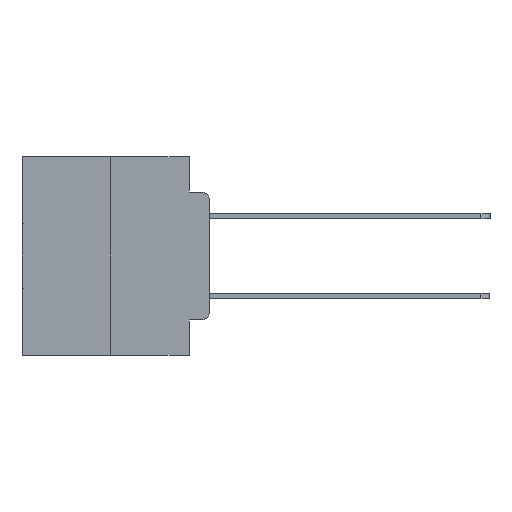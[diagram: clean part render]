
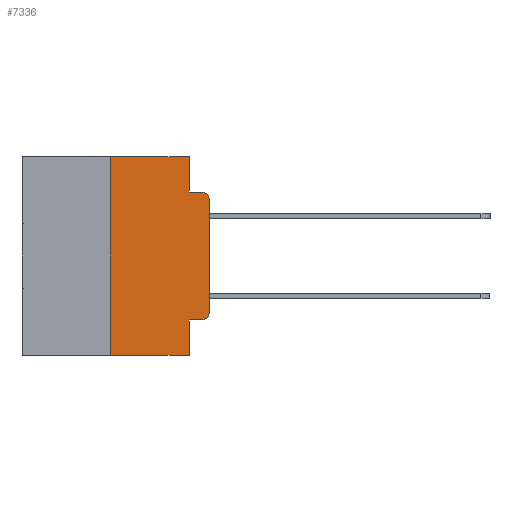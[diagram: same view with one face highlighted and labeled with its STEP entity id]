
A CAD part, left-side view. The second image highlights one B-rep face of the part: STEP entity #7336.
In plain terms, the highlighted planar face has unit normal (-1, 0, 0).
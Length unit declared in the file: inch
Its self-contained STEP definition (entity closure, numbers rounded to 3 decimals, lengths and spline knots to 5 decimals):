
#680 = CARTESIAN_POINT ( 'NONE',  ( 0., 0., -0.3915 ) ) ;
#836 = EDGE_CURVE ( 'NONE', #3411, #23348, #25860, .T. ) ;
#1466 = VECTOR ( 'NONE', #19686, 39.37008 ) ;
#1723 = ORIENTED_EDGE ( 'NONE', *, *, #10384, .T. ) ;
#2274 = EDGE_CURVE ( 'NONE', #13589, #26955, #28338, .T. ) ;
#2827 = CARTESIAN_POINT ( 'NONE',  ( 0., 0.051, 0. ) ) ;
#3411 = VERTEX_POINT ( 'NONE', #680 ) ;
#3655 = CARTESIAN_POINT ( 'NONE',  ( 0., 0.051, 0. ) ) ;
#3958 = CARTESIAN_POINT ( 'NONE',  ( 0., 0.051, -0.4115 ) ) ;
#4455 = DIRECTION ( 'NONE',  ( 0., 0., 1. ) ) ;
#5189 = DIRECTION ( 'NONE',  ( 0., 0., -1. ) ) ;
#5257 = CARTESIAN_POINT ( 'NONE',  ( 0., 0.051, 0. ) ) ;
#5335 = EDGE_CURVE ( 'NONE', #13589, #10760, #19099, .T. ) ;
#5661 = VECTOR ( 'NONE', #10762, 39.37008 ) ;
#5705 = CARTESIAN_POINT ( 'NONE',  ( 0., 0.051, -0.4115 ) ) ;
#6763 = EDGE_LOOP ( 'NONE', ( #10956, #25575, #13891, #9079, #10592, #19781, #1723, #22720, #28891, #23446 ) ) ;
#7017 = VECTOR ( 'NONE', #26369, 39.37008 ) ;
#7336 = ADVANCED_FACE ( 'NONE', ( #27312 ), #27479, .F. ) ;
#7670 = EDGE_CURVE ( 'NONE', #22380, #28418, #8952, .T. ) ;
#8102 = CARTESIAN_POINT ( 'NONE',  ( 0., 0.051, -0.0885 ) ) ;
#8650 = AXIS2_PLACEMENT_3D ( 'NONE', #10278, #26633, #12661 ) ;
#8952 = LINE ( 'NONE', #2827, #24745 ) ;
#9079 = ORIENTED_EDGE ( 'NONE', *, *, #7670, .F. ) ;
#9425 = LINE ( 'NONE', #26727, #21212 ) ;
#10012 = CARTESIAN_POINT ( 'NONE',  ( 0., 0.051, -0.0885 ) ) ;
#10278 = CARTESIAN_POINT ( 'NONE',  ( 0., 0.02, -0.3915 ) ) ;
#10384 = EDGE_CURVE ( 'NONE', #14808, #26955, #30435, .T. ) ;
#10592 = ORIENTED_EDGE ( 'NONE', *, *, #23770, .F. ) ;
#10760 = VERTEX_POINT ( 'NONE', #23239 ) ;
#10762 = DIRECTION ( 'NONE',  ( 0., 0., 1. ) ) ;
#10799 = CARTESIAN_POINT ( 'NONE',  ( 0., 0., 0. ) ) ;
#10898 = DIRECTION ( 'NONE',  ( -1., 0., 0. ) ) ;
#10956 = ORIENTED_EDGE ( 'NONE', *, *, #836, .T. ) ;
#11226 = CIRCLE ( 'NONE', #11495, 0.02 ) ;
#11495 = AXIS2_PLACEMENT_3D ( 'NONE', #24898, #10898, #27248 ) ;
#11972 = CIRCLE ( 'NONE', #8650, 0.02 ) ;
#12661 = DIRECTION ( 'NONE',  ( 0., 0., -1. ) ) ;
#12873 = DIRECTION ( 'NONE',  ( 0., -1., 0. ) ) ;
#13069 = DIRECTION ( 'NONE',  ( 0., 0., -1. ) ) ;
#13190 = VERTEX_POINT ( 'NONE', #19035 ) ;
#13377 = EDGE_CURVE ( 'NONE', #10760, #3411, #11972, .T. ) ;
#13499 = DIRECTION ( 'NONE',  ( 1., 0., 0. ) ) ;
#13589 = VERTEX_POINT ( 'NONE', #3958 ) ;
#13891 = ORIENTED_EDGE ( 'NONE', *, *, #19789, .F. ) ;
#14808 = VERTEX_POINT ( 'NONE', #27583 ) ;
#15757 = LINE ( 'NONE', #30170, #27422 ) ;
#17352 = CARTESIAN_POINT ( 'NONE',  ( 0., 0.473, -0.5 ) ) ;
#18360 = VECTOR ( 'NONE', #12873, 39.37008 ) ;
#19035 = CARTESIAN_POINT ( 'NONE',  ( 0., 0.25, 0. ) ) ;
#19099 = LINE ( 'NONE', #5705, #18360 ) ;
#19318 = VERTEX_POINT ( 'NONE', #24175 ) ;
#19686 = DIRECTION ( 'NONE',  ( 0., -1., 0. ) ) ;
#19781 = ORIENTED_EDGE ( 'NONE', *, *, #26858, .F. ) ;
#19789 = EDGE_CURVE ( 'NONE', #28418, #19318, #25033, .T. ) ;
#21212 = VECTOR ( 'NONE', #29068, 39.37008 ) ;
#21262 = CARTESIAN_POINT ( 'NONE',  ( 0., 0.051, -0.5 ) ) ;
#21393 = AXIS2_PLACEMENT_3D ( 'NONE', #22817, #13499, #29792 ) ;
#22380 = VERTEX_POINT ( 'NONE', #5257 ) ;
#22720 = ORIENTED_EDGE ( 'NONE', *, *, #2274, .F. ) ;
#22817 = CARTESIAN_POINT ( 'NONE',  ( 0., 0.473, 0. ) ) ;
#23239 = CARTESIAN_POINT ( 'NONE',  ( 0., 0.02, -0.4115 ) ) ;
#23348 = VERTEX_POINT ( 'NONE', #29692 ) ;
#23446 = ORIENTED_EDGE ( 'NONE', *, *, #13377, .T. ) ;
#23770 = EDGE_CURVE ( 'NONE', #13190, #22380, #9425, .T. ) ;
#24175 = CARTESIAN_POINT ( 'NONE',  ( 0., 0.02, -0.0885 ) ) ;
#24745 = VECTOR ( 'NONE', #5189, 39.37008 ) ;
#24867 = EDGE_CURVE ( 'NONE', #23348, #19318, #11226, .T. ) ;
#24898 = CARTESIAN_POINT ( 'NONE',  ( 0., 0.02, -0.1085 ) ) ;
#25033 = LINE ( 'NONE', #10012, #7017 ) ;
#25575 = ORIENTED_EDGE ( 'NONE', *, *, #24867, .T. ) ;
#25860 = LINE ( 'NONE', #10799, #5661 ) ;
#26369 = DIRECTION ( 'NONE',  ( 0., -1., 0. ) ) ;
#26633 = DIRECTION ( 'NONE',  ( -1., 0., 0. ) ) ;
#26727 = CARTESIAN_POINT ( 'NONE',  ( 0., 0.473, 0. ) ) ;
#26858 = EDGE_CURVE ( 'NONE', #14808, #13190, #15757, .T. ) ;
#26955 = VERTEX_POINT ( 'NONE', #21262 ) ;
#27248 = DIRECTION ( 'NONE',  ( 0., 0., -1. ) ) ;
#27312 = FACE_OUTER_BOUND ( 'NONE', #6763, .T. ) ;
#27422 = VECTOR ( 'NONE', #4455, 39.37008 ) ;
#27479 = PLANE ( 'NONE',  #21393 ) ;
#27583 = CARTESIAN_POINT ( 'NONE',  ( 0., 0.25, -0.5 ) ) ;
#27601 = VECTOR ( 'NONE', #13069, 39.37008 ) ;
#28338 = LINE ( 'NONE', #3655, #27601 ) ;
#28418 = VERTEX_POINT ( 'NONE', #8102 ) ;
#28891 = ORIENTED_EDGE ( 'NONE', *, *, #5335, .T. ) ;
#29068 = DIRECTION ( 'NONE',  ( 0., -1., 0. ) ) ;
#29692 = CARTESIAN_POINT ( 'NONE',  ( 0., 0., -0.1085 ) ) ;
#29792 = DIRECTION ( 'NONE',  ( 0., 0., -1. ) ) ;
#30170 = CARTESIAN_POINT ( 'NONE',  ( 0., 0.25, 0. ) ) ;
#30435 = LINE ( 'NONE', #17352, #1466 ) ;
